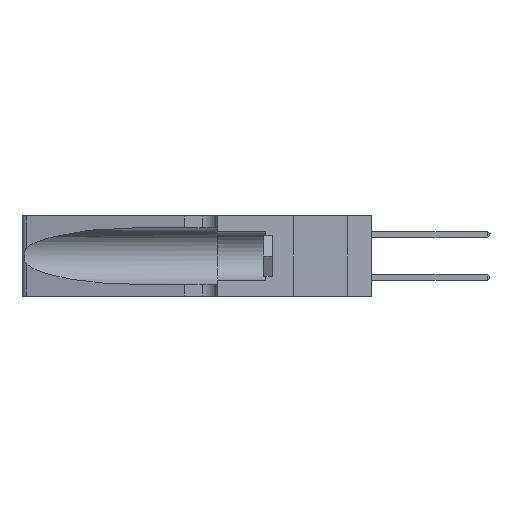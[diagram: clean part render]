
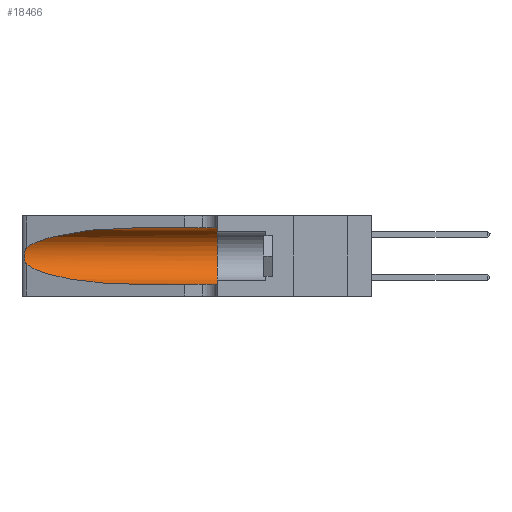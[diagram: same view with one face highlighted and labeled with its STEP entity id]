
A CAD part, left-side view. The second image highlights one B-rep face of the part: STEP entity #18466.
In plain terms, the highlighted cylindrical face has radius 3.308 mm (diameter 6.617 mm), a partial arc.
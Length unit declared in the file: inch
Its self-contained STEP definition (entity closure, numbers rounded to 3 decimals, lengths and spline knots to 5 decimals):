
#22 = VERTEX_POINT ( 'NONE', #4612 ) ;
#1033 = LINE ( 'NONE', #7423, #6181 ) ;
#1525 = CARTESIAN_POINT ( 'NONE',  ( 0.25487, 1.22718, 0.14631 ) ) ;
#1550 = DIRECTION ( 'NONE',  ( 0., -1., 0. ) ) ;
#1811 = ORIENTED_EDGE ( 'NONE', *, *, #8792, .F. ) ;
#2010 = ORIENTED_EDGE ( 'NONE', *, *, #2729, .T. ) ;
#2285 = CARTESIAN_POINT ( 'NONE',  ( 0.1305, 0.35, 0.05475 ) ) ;
#2364 = VERTEX_POINT ( 'NONE', #11372 ) ;
#2549 = CARTESIAN_POINT ( 'NONE',  ( 0.1305, 0.72297, 0.05475 ) ) ;
#2729 = EDGE_CURVE ( 'NONE', #21776, #10854, #1033, .T. ) ;
#3132 =( BOUNDED_CURVE ( )  B_SPLINE_CURVE ( 3, ( #16636, #14521, #10478, #24005 ),
 .UNSPECIFIED., .F., .T. ) 
 B_SPLINE_CURVE_WITH_KNOTS ( ( 4, 4 ),
 ( 3.44316, 4.71239 ),
 .UNSPECIFIED. ) 
 CURVE ( )  GEOMETRIC_REPRESENTATION_ITEM ( )  RATIONAL_B_SPLINE_CURVE ( ( 1., 0.87, 0.87, 1. ) ) 
 REPRESENTATION_ITEM ( '' )  );
#3601 = CARTESIAN_POINT ( 'NONE',  ( 0.25487, 1.22718, 0.22369 ) ) ;
#3677 = CARTESIAN_POINT ( 'NONE',  ( 0.25555, 1.22993, 0.14849 ) ) ;
#4535 = AXIS2_PLACEMENT_3D ( 'NONE', #17930, #23488, #13917 ) ;
#4612 = CARTESIAN_POINT ( 'NONE',  ( 0.25487, 1.22718, 0.22369 ) ) ;
#5501 = CARTESIAN_POINT ( 'NONE',  ( 0.1305, 0.72297, 0.31525 ) ) ;
#6181 = VECTOR ( 'NONE', #16032, 39.37008 ) ;
#6653 = ORIENTED_EDGE ( 'NONE', *, *, #7073, .T. ) ;
#6755 = EDGE_LOOP ( 'NONE', ( #10685, #14632, #6653, #2010, #20860, #1811 ) ) ;
#7045 = DIRECTION ( 'NONE',  ( 0., 0., -1. ) ) ;
#7073 = EDGE_CURVE ( 'NONE', #19178, #21776, #3132, .T. ) ;
#7202 = CARTESIAN_POINT ( 'NONE',  ( 0.18966, 0.96281, 0.31525 ) ) ;
#7360 = CARTESIAN_POINT ( 'NONE',  ( 0.25487, 1.22718, 0.22369 ) ) ;
#7373 = CARTESIAN_POINT ( 'NONE',  ( 0.1305, 1.61858, 0.185 ) ) ;
#7423 = CARTESIAN_POINT ( 'NONE',  ( 0.1305, 1.61858, 0.05475 ) ) ;
#8792 = EDGE_CURVE ( 'NONE', #2364, #11209, #20307, .T. ) ;
#9065 = CARTESIAN_POINT ( 'NONE',  ( 0.1305, 1.61858, 0.31525 ) ) ;
#9259 = CARTESIAN_POINT ( 'NONE',  ( 0.26075, 1.23896, 0.178 ) ) ;
#9416 = CARTESIAN_POINT ( 'NONE',  ( 0.25555, 1.22994, 0.2215 ) ) ;
#9733 = FACE_OUTER_BOUND ( 'NONE', #6755, .T. ) ;
#9808 = CARTESIAN_POINT ( 'NONE',  ( 0.25487, 1.22718, 0.14631 ) ) ;
#10201 = B_SPLINE_CURVE_WITH_KNOTS ( 'NONE', 3,
 ( #3601, #9416, #22838, #11153, #21319, #13187, #23341, #9259, #20846, #19079, #11812, #18923, #3677, #9808 ),
 .UNSPECIFIED., .F., .F.,
 ( 4, 2, 2, 2, 2, 2, 4 ),
 ( 0., 0.00027, 0.00053, 0.00107, 0.0016, 0.00187, 0.00214 ),
 .UNSPECIFIED. ) ;
#10478 = CARTESIAN_POINT ( 'NONE',  ( 0.18966, 0.96281, 0.05475 ) ) ;
#10685 = ORIENTED_EDGE ( 'NONE', *, *, #20246, .T. ) ;
#10854 = VERTEX_POINT ( 'NONE', #2285 ) ;
#11153 = CARTESIAN_POINT ( 'NONE',  ( 0.25787, 1.23484, 0.2124 ) ) ;
#11209 = VERTEX_POINT ( 'NONE', #14170 ) ;
#11372 = CARTESIAN_POINT ( 'NONE',  ( 0.1305, 0.72297, 0.31525 ) ) ;
#11812 = CARTESIAN_POINT ( 'NONE',  ( 0.25789, 1.23486, 0.15765 ) ) ;
#12128 = CYLINDRICAL_SURFACE ( 'NONE', #16011, 0.13025 ) ;
#12479 = VECTOR ( 'NONE', #19217, 39.37008 ) ;
#13187 = CARTESIAN_POINT ( 'NONE',  ( 0.26018, 1.23835, 0.19895 ) ) ;
#13225 = CIRCLE ( 'NONE', #4535, 0.13025 ) ;
#13917 = DIRECTION ( 'NONE',  ( 0., 0., 1. ) ) ;
#14170 = CARTESIAN_POINT ( 'NONE',  ( 0.1305, 0.35, 0.31525 ) ) ;
#14521 = CARTESIAN_POINT ( 'NONE',  ( 0.2373, 1.15595, 0.08982 ) ) ;
#14632 = ORIENTED_EDGE ( 'NONE', *, *, #24309, .T. ) ;
#14858 = EDGE_CURVE ( 'NONE', #11209, #10854, #13225, .T. ) ;
#16011 = AXIS2_PLACEMENT_3D ( 'NONE', #7373, #1550, #7045 ) ;
#16032 = DIRECTION ( 'NONE',  ( 0., -1., 0. ) ) ;
#16636 = CARTESIAN_POINT ( 'NONE',  ( 0.25487, 1.22718, 0.14631 ) ) ;
#17930 = CARTESIAN_POINT ( 'NONE',  ( 0.1305, 0.35, 0.185 ) ) ;
#18466 = ADVANCED_FACE ( 'NONE', ( #9733 ), #12128, .F. ) ;
#18892 = CARTESIAN_POINT ( 'NONE',  ( 0.2373, 1.15595, 0.28018 ) ) ;
#18923 = CARTESIAN_POINT ( 'NONE',  ( 0.25639, 1.23186, 0.15144 ) ) ;
#19079 = CARTESIAN_POINT ( 'NONE',  ( 0.25856, 1.23593, 0.16098 ) ) ;
#19178 = VERTEX_POINT ( 'NONE', #1525 ) ;
#19217 = DIRECTION ( 'NONE',  ( 0., -1., 0. ) ) ;
#20246 = EDGE_CURVE ( 'NONE', #2364, #22, #24070, .T. ) ;
#20307 = LINE ( 'NONE', #9065, #12479 ) ;
#20846 = CARTESIAN_POINT ( 'NONE',  ( 0.26017, 1.23833, 0.17102 ) ) ;
#20860 = ORIENTED_EDGE ( 'NONE', *, *, #14858, .F. ) ;
#21319 = CARTESIAN_POINT ( 'NONE',  ( 0.25854, 1.2359, 0.20912 ) ) ;
#21776 = VERTEX_POINT ( 'NONE', #2549 ) ;
#22838 = CARTESIAN_POINT ( 'NONE',  ( 0.25639, 1.23184, 0.21858 ) ) ;
#23341 = CARTESIAN_POINT ( 'NONE',  ( 0.26075, 1.23896, 0.19203 ) ) ;
#23488 = DIRECTION ( 'NONE',  ( 0., 1., 0. ) ) ;
#24005 = CARTESIAN_POINT ( 'NONE',  ( 0.1305, 0.72297, 0.05475 ) ) ;
#24070 =( BOUNDED_CURVE ( )  B_SPLINE_CURVE ( 3, ( #5501, #7202, #18892, #7360 ),
 .UNSPECIFIED., .F., .T. ) 
 B_SPLINE_CURVE_WITH_KNOTS ( ( 4, 4 ),
 ( 1.5708, 2.84003 ),
 .UNSPECIFIED. ) 
 CURVE ( )  GEOMETRIC_REPRESENTATION_ITEM ( )  RATIONAL_B_SPLINE_CURVE ( ( 1., 0.87, 0.87, 1. ) ) 
 REPRESENTATION_ITEM ( '' )  );
#24309 = EDGE_CURVE ( 'NONE', #22, #19178, #10201, .T. ) ;
